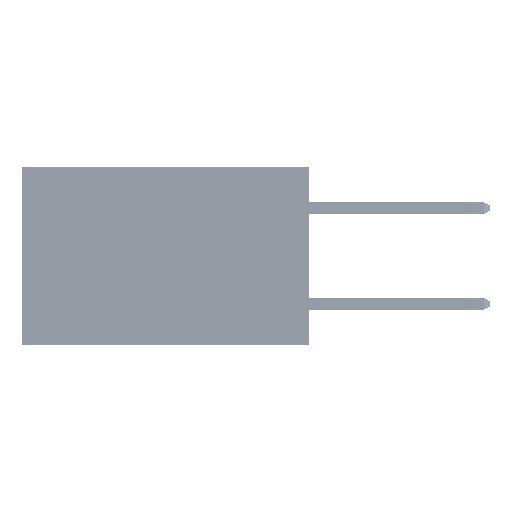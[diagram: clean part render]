
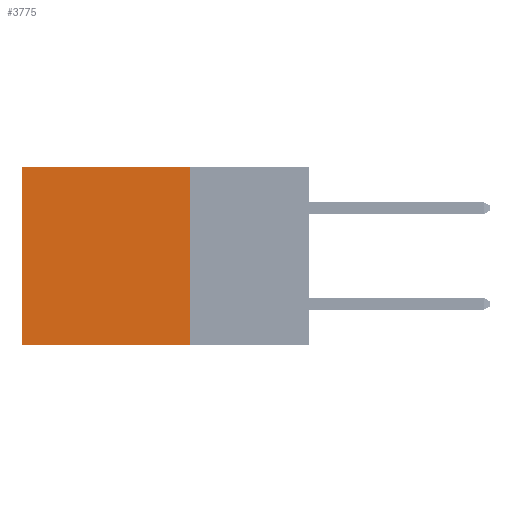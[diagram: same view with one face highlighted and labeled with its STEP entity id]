
A CAD part, left-side view. The second image highlights one B-rep face of the part: STEP entity #3775.
In plain terms, the highlighted planar face has unit normal (-1, 0, 0).
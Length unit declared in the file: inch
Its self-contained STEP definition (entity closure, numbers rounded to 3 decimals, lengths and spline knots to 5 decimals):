
#589 = ORIENTED_EDGE ( 'NONE', *, *, #15428, .T. ) ;
#1100 = EDGE_CURVE ( 'NONE', #16136, #40867, #19968, .T. ) ;
#1140 = VECTOR ( 'NONE', #5499, 39.37008 ) ;
#3526 = CARTESIAN_POINT ( 'NONE',  ( 0.2875, 0.6, -0.37 ) ) ;
#3775 = ADVANCED_FACE ( 'NONE', ( #30101 ), #19563, .F. ) ;
#4614 = LINE ( 'NONE', #38027, #37926 ) ;
#4857 = CARTESIAN_POINT ( 'NONE',  ( 0.2875, 0.25, 0. ) ) ;
#5499 = DIRECTION ( 'NONE',  ( 0., 0., -1. ) ) ;
#6854 = ORIENTED_EDGE ( 'NONE', *, *, #18095, .F. ) ;
#7515 = CARTESIAN_POINT ( 'NONE',  ( 0.2875, 0.25, 0. ) ) ;
#7635 = LINE ( 'NONE', #22250, #36624 ) ;
#9809 = VERTEX_POINT ( 'NONE', #31532 ) ;
#10047 = CARTESIAN_POINT ( 'NONE',  ( 0.2875, 0.25, -0.37 ) ) ;
#11822 = DIRECTION ( 'NONE',  ( 1., 0., 0. ) ) ;
#14704 = LINE ( 'NONE', #21182, #1140 ) ;
#15428 = EDGE_CURVE ( 'NONE', #9809, #40867, #14704, .T. ) ;
#16136 = VERTEX_POINT ( 'NONE', #39956 ) ;
#16294 = VECTOR ( 'NONE', #29857, 39.37008 ) ;
#18095 = EDGE_CURVE ( 'NONE', #40999, #16136, #7635, .T. ) ;
#19563 = PLANE ( 'NONE',  #32297 ) ;
#19968 = LINE ( 'NONE', #10047, #16294 ) ;
#20193 = EDGE_LOOP ( 'NONE', ( #589, #37395, #6854, #29966 ) ) ;
#21182 = CARTESIAN_POINT ( 'NONE',  ( 0.2875, 0.6, 0. ) ) ;
#21507 = EDGE_CURVE ( 'NONE', #40999, #9809, #4614, .T. ) ;
#22250 = CARTESIAN_POINT ( 'NONE',  ( 0.2875, 0.25, 0. ) ) ;
#29857 = DIRECTION ( 'NONE',  ( 0., 1., 0. ) ) ;
#29966 = ORIENTED_EDGE ( 'NONE', *, *, #21507, .T. ) ;
#30101 = FACE_OUTER_BOUND ( 'NONE', #20193, .T. ) ;
#31532 = CARTESIAN_POINT ( 'NONE',  ( 0.2875, 0.6, 0. ) ) ;
#32297 = AXIS2_PLACEMENT_3D ( 'NONE', #7515, #11822, #35101 ) ;
#34165 = DIRECTION ( 'NONE',  ( 0., 0., -1. ) ) ;
#34723 = DIRECTION ( 'NONE',  ( 0., 1., 0. ) ) ;
#35101 = DIRECTION ( 'NONE',  ( 0., 0., -1. ) ) ;
#36624 = VECTOR ( 'NONE', #34165, 39.37008 ) ;
#37395 = ORIENTED_EDGE ( 'NONE', *, *, #1100, .F. ) ;
#37926 = VECTOR ( 'NONE', #34723, 39.37008 ) ;
#38027 = CARTESIAN_POINT ( 'NONE',  ( 0.2875, 0.25, 0. ) ) ;
#39956 = CARTESIAN_POINT ( 'NONE',  ( 0.2875, 0.25, -0.37 ) ) ;
#40867 = VERTEX_POINT ( 'NONE', #3526 ) ;
#40999 = VERTEX_POINT ( 'NONE', #4857 ) ;
